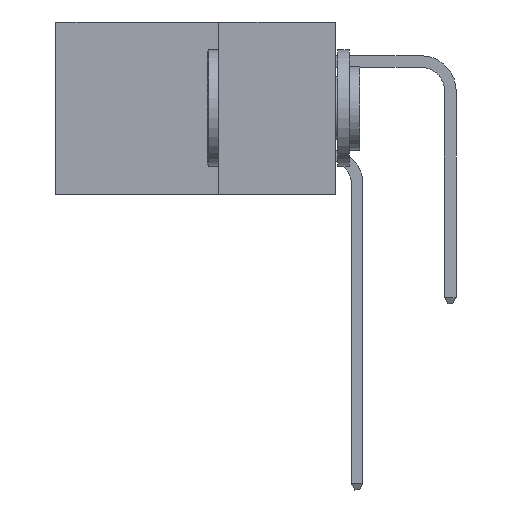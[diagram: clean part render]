
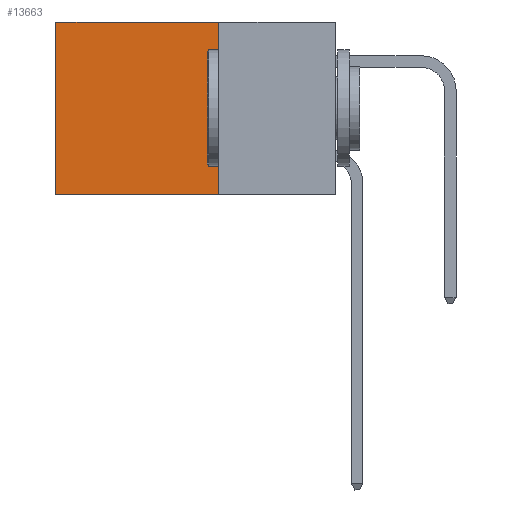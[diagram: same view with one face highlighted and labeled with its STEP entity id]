
A CAD part, left-side view. The second image highlights one B-rep face of the part: STEP entity #13663.
In plain terms, the highlighted planar face has unit normal (-1, 0, 0).
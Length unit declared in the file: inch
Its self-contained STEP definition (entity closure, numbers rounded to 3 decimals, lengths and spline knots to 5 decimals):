
#51 = EDGE_CURVE ( 'NONE', #9389, #5996, #2396, .T. ) ;
#220 = DIRECTION ( 'NONE',  ( 1., 0., 0. ) ) ;
#618 = DIRECTION ( 'NONE',  ( 0., 1., 0. ) ) ;
#1857 = CARTESIAN_POINT ( 'NONE',  ( 0.2875, 0.25, 0. ) ) ;
#2049 = EDGE_LOOP ( 'NONE', ( #4916, #2421, #13028, #18600 ) ) ;
#2396 = LINE ( 'NONE', #3341, #15056 ) ;
#2421 = ORIENTED_EDGE ( 'NONE', *, *, #12157, .F. ) ;
#2803 = DIRECTION ( 'NONE',  ( 0., 0., -1. ) ) ;
#3341 = CARTESIAN_POINT ( 'NONE',  ( 0.2875, 0.6, 0. ) ) ;
#4670 = FACE_OUTER_BOUND ( 'NONE', #2049, .T. ) ;
#4916 = ORIENTED_EDGE ( 'NONE', *, *, #51, .T. ) ;
#5288 = VERTEX_POINT ( 'NONE', #6446 ) ;
#5996 = VERTEX_POINT ( 'NONE', #19476 ) ;
#6393 = EDGE_CURVE ( 'NONE', #15553, #5288, #11539, .T. ) ;
#6446 = CARTESIAN_POINT ( 'NONE',  ( 0.2875, 0.25, -0.37 ) ) ;
#6873 = LINE ( 'NONE', #9372, #17111 ) ;
#7487 = DIRECTION ( 'NONE',  ( 0., 0., -1. ) ) ;
#8027 = DIRECTION ( 'NONE',  ( 0., 0., -1. ) ) ;
#9092 = VECTOR ( 'NONE', #2803, 39.37008 ) ;
#9217 = DIRECTION ( 'NONE',  ( 0., 1., 0. ) ) ;
#9372 = CARTESIAN_POINT ( 'NONE',  ( 0.2875, 0.25, 0. ) ) ;
#9389 = VERTEX_POINT ( 'NONE', #11504 ) ;
#10918 = CARTESIAN_POINT ( 'NONE',  ( 0.2875, 0.25, -0.37 ) ) ;
#11234 = AXIS2_PLACEMENT_3D ( 'NONE', #16452, #220, #8027 ) ;
#11504 = CARTESIAN_POINT ( 'NONE',  ( 0.2875, 0.6, 0. ) ) ;
#11539 = LINE ( 'NONE', #21640, #9092 ) ;
#12157 = EDGE_CURVE ( 'NONE', #5288, #5996, #16843, .T. ) ;
#13028 = ORIENTED_EDGE ( 'NONE', *, *, #6393, .F. ) ;
#13663 = ADVANCED_FACE ( 'NONE', ( #4670 ), #15990, .F. ) ;
#15056 = VECTOR ( 'NONE', #7487, 39.37008 ) ;
#15553 = VERTEX_POINT ( 'NONE', #1857 ) ;
#15990 = PLANE ( 'NONE',  #11234 ) ;
#15994 = VECTOR ( 'NONE', #618, 39.37008 ) ;
#16452 = CARTESIAN_POINT ( 'NONE',  ( 0.2875, 0.25, 0. ) ) ;
#16843 = LINE ( 'NONE', #10918, #15994 ) ;
#17111 = VECTOR ( 'NONE', #9217, 39.37008 ) ;
#18600 = ORIENTED_EDGE ( 'NONE', *, *, #21438, .T. ) ;
#19476 = CARTESIAN_POINT ( 'NONE',  ( 0.2875, 0.6, -0.37 ) ) ;
#21438 = EDGE_CURVE ( 'NONE', #15553, #9389, #6873, .T. ) ;
#21640 = CARTESIAN_POINT ( 'NONE',  ( 0.2875, 0.25, 0. ) ) ;
